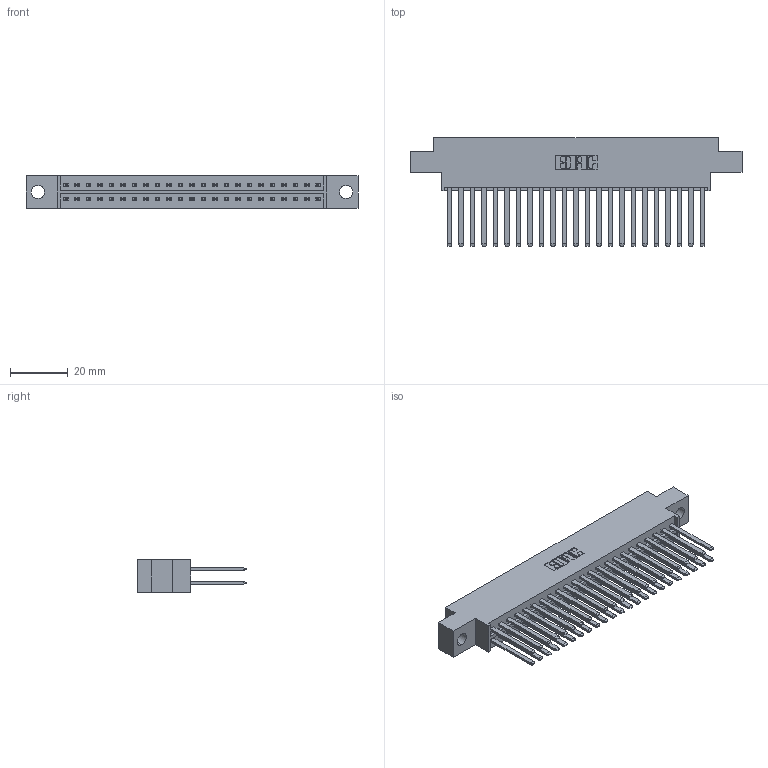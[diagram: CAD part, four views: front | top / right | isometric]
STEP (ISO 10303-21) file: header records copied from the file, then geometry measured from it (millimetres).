
FILE_DESCRIPTION (( 'STEP AP203' ), '1' );
FILE_NAME ('336-046-541-809.STEP', '2020-08-08T00:00:04', ( '' ), ( '' ), 'SwSTEP 2.0', 'SolidWorks 2020', '' );
FILE_SCHEMA (( 'CONFIG_CONTROL_DESIGN' ));
Length unit declared in the file: inch
Products named in the file (3): 336-290-001_336-290-541; 336 Part_Offset - .178 Dia - TH; 336-046-541-809
Assembly tree (47 placements, depth 2):
  336-046-541-809
    336 Part_Offset - .178 Dia - TH
    336-290-001_336-290-541  x46
Bounding box: 114.53 x 37.34 x 11.1 mm (x, y, z)
Volume: 16928 mm3; surface area: 21236.2 mm2
Topology: 47 solids, 47 shells, 2050 faces, 6165 edges, 4078 vertices
Faces by surface type: plane 1270, cylinder 780
Entity records: 20144 total; most frequent: CARTESIAN_POINT 3493, ORIENTED_EDGE 3330, DIRECTION 2909, EDGE_CURVE 1665, LINE 1533, VECTOR 1533, VERTEX_POINT 1108, AXIS2_PLACEMENT_3D 688
